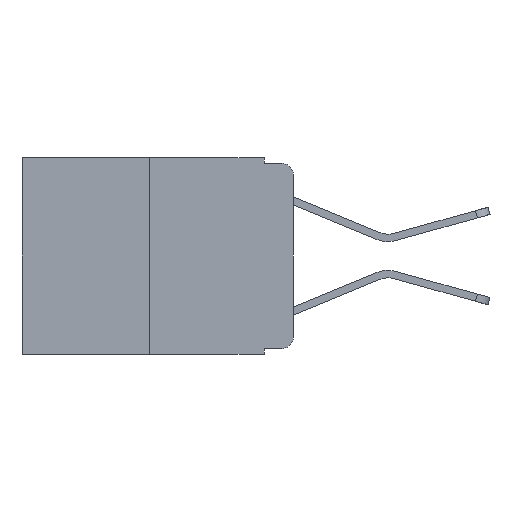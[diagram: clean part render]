
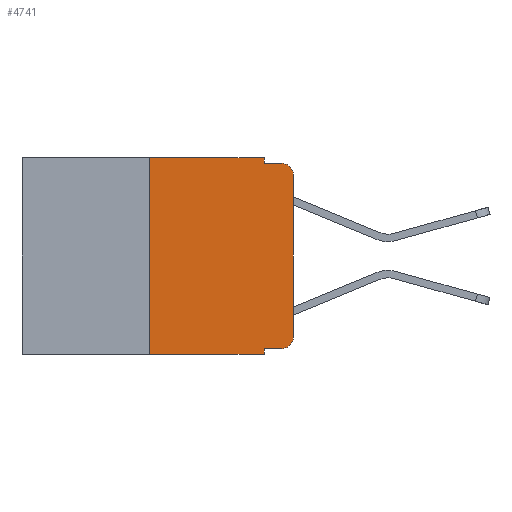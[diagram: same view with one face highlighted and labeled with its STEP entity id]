
A CAD part, left-side view. The second image highlights one B-rep face of the part: STEP entity #4741.
In plain terms, the highlighted planar face has unit normal (-1, 0, 0).
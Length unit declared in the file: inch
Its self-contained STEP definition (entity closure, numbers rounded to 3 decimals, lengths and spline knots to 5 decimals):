
#97 = ORIENTED_EDGE ( 'NONE', *, *, #8975, .T. ) ;
#466 = EDGE_CURVE ( 'NONE', #1737, #9706, #6524, .T. ) ;
#503 = DIRECTION ( 'NONE',  ( -1., 0., 0. ) ) ;
#528 = VECTOR ( 'NONE', #4911, 39.37008 ) ;
#545 = ORIENTED_EDGE ( 'NONE', *, *, #5131, .F. ) ;
#794 = CARTESIAN_POINT ( 'NONE',  ( 0., 0.473, 0. ) ) ;
#1054 = ORIENTED_EDGE ( 'NONE', *, *, #1930, .F. ) ;
#1087 = DIRECTION ( 'NONE',  ( 1., 0., 0. ) ) ;
#1166 = VECTOR ( 'NONE', #9757, 39.37008 ) ;
#1243 = CARTESIAN_POINT ( 'NONE',  ( 0., 0.02, -0.01 ) ) ;
#1248 = DIRECTION ( 'NONE',  ( 0., 0., -1. ) ) ;
#1293 = CARTESIAN_POINT ( 'NONE',  ( 0., 0.051, 0. ) ) ;
#1294 = VECTOR ( 'NONE', #4595, 39.37008 ) ;
#1505 = CARTESIAN_POINT ( 'NONE',  ( 0., 0.02, -0.313 ) ) ;
#1737 = VERTEX_POINT ( 'NONE', #2258 ) ;
#1740 = VERTEX_POINT ( 'NONE', #9944 ) ;
#1802 = EDGE_LOOP ( 'NONE', ( #8371, #4392, #545, #4622, #1054, #5950, #6219, #7591, #7952, #97 ) ) ;
#1825 = CARTESIAN_POINT ( 'NONE',  ( 0., 0.25, 0. ) ) ;
#1886 = VERTEX_POINT ( 'NONE', #9246 ) ;
#1930 = EDGE_CURVE ( 'NONE', #3322, #2676, #6237, .T. ) ;
#2198 = VECTOR ( 'NONE', #9353, 39.37008 ) ;
#2258 = CARTESIAN_POINT ( 'NONE',  ( 0., 0.051, -0.333 ) ) ;
#2270 = DIRECTION ( 'NONE',  ( 0., 0., -1. ) ) ;
#2349 = DIRECTION ( 'NONE',  ( 0., 0., -1. ) ) ;
#2635 = CARTESIAN_POINT ( 'NONE',  ( 0., 0.051, 0. ) ) ;
#2639 = DIRECTION ( 'NONE',  ( 0., -1., 0. ) ) ;
#2676 = VERTEX_POINT ( 'NONE', #9830 ) ;
#3322 = VERTEX_POINT ( 'NONE', #1825 ) ;
#3584 = AXIS2_PLACEMENT_3D ( 'NONE', #794, #1087, #2270 ) ;
#3794 = EDGE_CURVE ( 'NONE', #1737, #5861, #8879, .T. ) ;
#3955 = VECTOR ( 'NONE', #8866, 39.37008 ) ;
#4392 = ORIENTED_EDGE ( 'NONE', *, *, #8893, .T. ) ;
#4412 = CARTESIAN_POINT ( 'NONE',  ( 0., 0., -0.313 ) ) ;
#4549 = CARTESIAN_POINT ( 'NONE',  ( 0., 0.051, -0.333 ) ) ;
#4595 = DIRECTION ( 'NONE',  ( 0., 0., 1. ) ) ;
#4622 = ORIENTED_EDGE ( 'NONE', *, *, #8227, .F. ) ;
#4741 = ADVANCED_FACE ( 'NONE', ( #6750 ), #5480, .F. ) ;
#4878 = EDGE_CURVE ( 'NONE', #6066, #1886, #9628, .T. ) ;
#4911 = DIRECTION ( 'NONE',  ( 0., 0., -1. ) ) ;
#4920 = CARTESIAN_POINT ( 'NONE',  ( 0., 0.051, -0.01 ) ) ;
#4944 = VECTOR ( 'NONE', #1248, 39.37008 ) ;
#4950 = CARTESIAN_POINT ( 'NONE',  ( 0., 0.051, -0.343 ) ) ;
#5131 = EDGE_CURVE ( 'NONE', #5845, #9887, #8849, .T. ) ;
#5220 = EDGE_CURVE ( 'NONE', #1740, #5861, #7990, .T. ) ;
#5319 = DIRECTION ( 'NONE',  ( 0., -1., 0. ) ) ;
#5335 = CARTESIAN_POINT ( 'NONE',  ( 0., 0.02, -0.03 ) ) ;
#5458 = AXIS2_PLACEMENT_3D ( 'NONE', #5335, #503, #6107 ) ;
#5480 = PLANE ( 'NONE',  #3584 ) ;
#5845 = VERTEX_POINT ( 'NONE', #4920 ) ;
#5857 = EDGE_CURVE ( 'NONE', #1740, #3322, #8305, .T. ) ;
#5861 = VERTEX_POINT ( 'NONE', #4950 ) ;
#5950 = ORIENTED_EDGE ( 'NONE', *, *, #5857, .F. ) ;
#6066 = VERTEX_POINT ( 'NONE', #4412 ) ;
#6107 = DIRECTION ( 'NONE',  ( 0., 0., -1. ) ) ;
#6219 = ORIENTED_EDGE ( 'NONE', *, *, #5220, .T. ) ;
#6237 = LINE ( 'NONE', #8735, #3955 ) ;
#6271 = VECTOR ( 'NONE', #2639, 39.37008 ) ;
#6524 = LINE ( 'NONE', #4549, #6271 ) ;
#6674 = LINE ( 'NONE', #2635, #528 ) ;
#6750 = FACE_OUTER_BOUND ( 'NONE', #1802, .T. ) ;
#7010 = DIRECTION ( 'NONE',  ( -1., 0., 0. ) ) ;
#7403 = CARTESIAN_POINT ( 'NONE',  ( 0., 0.473, -0.343 ) ) ;
#7451 = CARTESIAN_POINT ( 'NONE',  ( 0., 0., 0. ) ) ;
#7488 = CIRCLE ( 'NONE', #5458, 0.02 ) ;
#7591 = ORIENTED_EDGE ( 'NONE', *, *, #3794, .F. ) ;
#7952 = ORIENTED_EDGE ( 'NONE', *, *, #466, .T. ) ;
#7989 = AXIS2_PLACEMENT_3D ( 'NONE', #1505, #7010, #2349 ) ;
#7990 = LINE ( 'NONE', #7403, #9826 ) ;
#7999 = CARTESIAN_POINT ( 'NONE',  ( 0., 0.02, -0.333 ) ) ;
#8227 = EDGE_CURVE ( 'NONE', #2676, #5845, #6674, .T. ) ;
#8305 = LINE ( 'NONE', #8643, #2198 ) ;
#8371 = ORIENTED_EDGE ( 'NONE', *, *, #4878, .T. ) ;
#8465 = CIRCLE ( 'NONE', #7989, 0.02 ) ;
#8467 = CARTESIAN_POINT ( 'NONE',  ( 0., 0.051, -0.01 ) ) ;
#8643 = CARTESIAN_POINT ( 'NONE',  ( 0., 0.25, 0. ) ) ;
#8735 = CARTESIAN_POINT ( 'NONE',  ( 0., 0.473, 0. ) ) ;
#8849 = LINE ( 'NONE', #8467, #1166 ) ;
#8866 = DIRECTION ( 'NONE',  ( 0., -1., 0. ) ) ;
#8879 = LINE ( 'NONE', #1293, #4944 ) ;
#8893 = EDGE_CURVE ( 'NONE', #1886, #9887, #7488, .T. ) ;
#8975 = EDGE_CURVE ( 'NONE', #9706, #6066, #8465, .T. ) ;
#9246 = CARTESIAN_POINT ( 'NONE',  ( 0., 0., -0.03 ) ) ;
#9353 = DIRECTION ( 'NONE',  ( 0., 0., 1. ) ) ;
#9628 = LINE ( 'NONE', #7451, #1294 ) ;
#9706 = VERTEX_POINT ( 'NONE', #7999 ) ;
#9757 = DIRECTION ( 'NONE',  ( 0., -1., 0. ) ) ;
#9826 = VECTOR ( 'NONE', #5319, 39.37008 ) ;
#9830 = CARTESIAN_POINT ( 'NONE',  ( 0., 0.051, 0. ) ) ;
#9887 = VERTEX_POINT ( 'NONE', #1243 ) ;
#9944 = CARTESIAN_POINT ( 'NONE',  ( 0., 0.25, -0.343 ) ) ;
